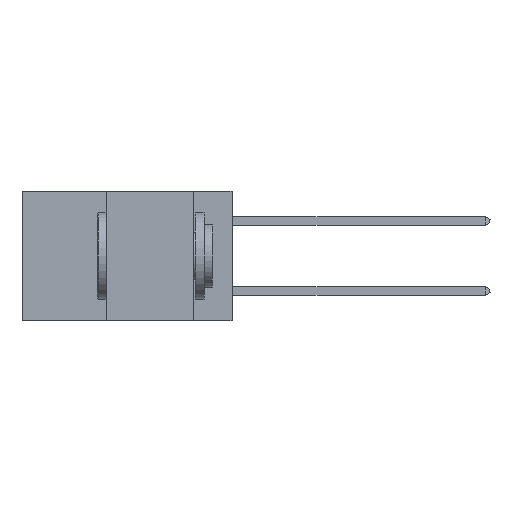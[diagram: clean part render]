
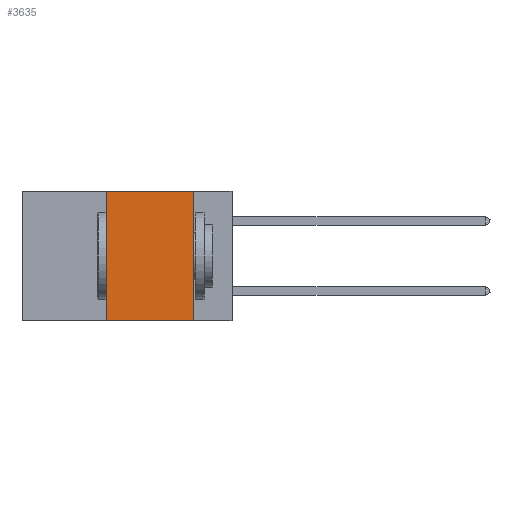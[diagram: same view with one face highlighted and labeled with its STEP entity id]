
A CAD part, left-side view. The second image highlights one B-rep face of the part: STEP entity #3635.
In plain terms, the highlighted planar face has unit normal (-1, 0, 0).
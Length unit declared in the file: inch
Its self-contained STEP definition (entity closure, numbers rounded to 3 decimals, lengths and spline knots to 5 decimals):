
#1484 = CARTESIAN_POINT ( 'NONE',  ( 0., 0.11, 0. ) ) ;
#3189 = FACE_OUTER_BOUND ( 'NONE', #15959, .T. ) ;
#3635 = ADVANCED_FACE ( 'NONE', ( #3189 ), #20130, .F. ) ;
#4554 = EDGE_CURVE ( 'NONE', #25503, #19410, #31566, .T. ) ;
#5371 = CARTESIAN_POINT ( 'NONE',  ( 0., 0.36, -0.37 ) ) ;
#6356 = ORIENTED_EDGE ( 'NONE', *, *, #9896, .F. ) ;
#7177 = CARTESIAN_POINT ( 'NONE',  ( 0., 0.36, 0. ) ) ;
#7379 = DIRECTION ( 'NONE',  ( 1., 0., 0. ) ) ;
#7509 = VERTEX_POINT ( 'NONE', #32031 ) ;
#8251 = CARTESIAN_POINT ( 'NONE',  ( 0., 0.6, -0.37 ) ) ;
#9576 = CARTESIAN_POINT ( 'NONE',  ( 0., 0.11, -0.37 ) ) ;
#9879 = DIRECTION ( 'NONE',  ( 0., 0., 1. ) ) ;
#9896 = EDGE_CURVE ( 'NONE', #28345, #7509, #11522, .T. ) ;
#10172 = ORIENTED_EDGE ( 'NONE', *, *, #23365, .F. ) ;
#10685 = VECTOR ( 'NONE', #14436, 39.37008 ) ;
#11522 = LINE ( 'NONE', #30640, #10685 ) ;
#14436 = DIRECTION ( 'NONE',  ( 0., -1., 0. ) ) ;
#15959 = EDGE_LOOP ( 'NONE', ( #30507, #6356, #10172, #18799 ) ) ;
#18149 = CARTESIAN_POINT ( 'NONE',  ( 0., 0.6, 0. ) ) ;
#18799 = ORIENTED_EDGE ( 'NONE', *, *, #4554, .T. ) ;
#19410 = VERTEX_POINT ( 'NONE', #9576 ) ;
#20130 = PLANE ( 'NONE',  #27566 ) ;
#20457 = DIRECTION ( 'NONE',  ( 0., 0., -1. ) ) ;
#22672 = CARTESIAN_POINT ( 'NONE',  ( 0., 0.36, 0. ) ) ;
#23365 = EDGE_CURVE ( 'NONE', #25503, #28345, #24575, .T. ) ;
#23528 = VECTOR ( 'NONE', #24464, 39.37008 ) ;
#24464 = DIRECTION ( 'NONE',  ( 0., -1., 0. ) ) ;
#24575 = LINE ( 'NONE', #7177, #30058 ) ;
#24638 = LINE ( 'NONE', #1484, #31811 ) ;
#25503 = VERTEX_POINT ( 'NONE', #5371 ) ;
#26277 = DIRECTION ( 'NONE',  ( 0., 0., -1. ) ) ;
#27566 = AXIS2_PLACEMENT_3D ( 'NONE', #18149, #7379, #26277 ) ;
#28345 = VERTEX_POINT ( 'NONE', #22672 ) ;
#30058 = VECTOR ( 'NONE', #9879, 39.37008 ) ;
#30507 = ORIENTED_EDGE ( 'NONE', *, *, #30617, .F. ) ;
#30617 = EDGE_CURVE ( 'NONE', #7509, #19410, #24638, .T. ) ;
#30640 = CARTESIAN_POINT ( 'NONE',  ( 0., 0.6, 0. ) ) ;
#31566 = LINE ( 'NONE', #8251, #23528 ) ;
#31811 = VECTOR ( 'NONE', #20457, 39.37008 ) ;
#32031 = CARTESIAN_POINT ( 'NONE',  ( 0., 0.11, 0. ) ) ;
